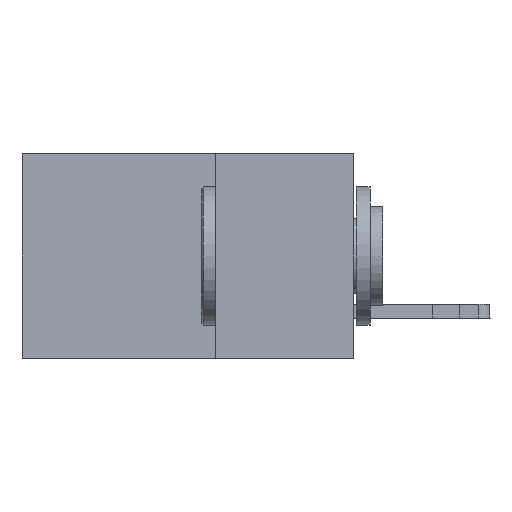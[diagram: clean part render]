
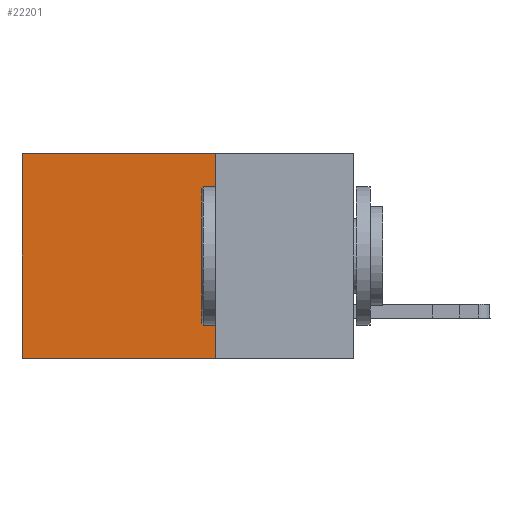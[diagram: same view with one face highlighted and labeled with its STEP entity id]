
A CAD part, left-side view. The second image highlights one B-rep face of the part: STEP entity #22201.
In plain terms, the highlighted planar face has unit normal (-1, 0, 0).
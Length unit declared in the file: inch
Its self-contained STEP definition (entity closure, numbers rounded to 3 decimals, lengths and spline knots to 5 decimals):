
#288 = DIRECTION ( 'NONE',  ( 0., 0., -1. ) ) ;
#457 = FACE_OUTER_BOUND ( 'NONE', #8507, .T. ) ;
#629 = LINE ( 'NONE', #10913, #10525 ) ;
#1062 = DIRECTION ( 'NONE',  ( 0., 0., -1. ) ) ;
#1547 = VERTEX_POINT ( 'NONE', #6921 ) ;
#2471 = ORIENTED_EDGE ( 'NONE', *, *, #16416, .F. ) ;
#4737 = DIRECTION ( 'NONE',  ( 0., 0., -1. ) ) ;
#6042 = EDGE_CURVE ( 'NONE', #14477, #6281, #6808, .T. ) ;
#6110 = CARTESIAN_POINT ( 'NONE',  ( 0.2875, 0.6, -0.37 ) ) ;
#6202 = VECTOR ( 'NONE', #288, 39.37008 ) ;
#6281 = VERTEX_POINT ( 'NONE', #16719 ) ;
#6305 = EDGE_CURVE ( 'NONE', #1547, #23799, #629, .T. ) ;
#6808 = LINE ( 'NONE', #19873, #6202 ) ;
#6815 = LINE ( 'NONE', #23169, #11470 ) ;
#6921 = CARTESIAN_POINT ( 'NONE',  ( 0.2875, 0.6, 0. ) ) ;
#7619 = LINE ( 'NONE', #21900, #17441 ) ;
#8507 = EDGE_LOOP ( 'NONE', ( #19367, #2471, #19189, #13010 ) ) ;
#10525 = VECTOR ( 'NONE', #1062, 39.37008 ) ;
#10913 = CARTESIAN_POINT ( 'NONE',  ( 0.2875, 0.6, 0. ) ) ;
#11470 = VECTOR ( 'NONE', #13450, 39.37008 ) ;
#12113 = DIRECTION ( 'NONE',  ( 0., 1., 0. ) ) ;
#13010 = ORIENTED_EDGE ( 'NONE', *, *, #20091, .T. ) ;
#13450 = DIRECTION ( 'NONE',  ( 0., 1., 0. ) ) ;
#14477 = VERTEX_POINT ( 'NONE', #16305 ) ;
#16305 = CARTESIAN_POINT ( 'NONE',  ( 0.2875, 0.25, 0. ) ) ;
#16416 = EDGE_CURVE ( 'NONE', #6281, #23799, #7619, .T. ) ;
#16514 = DIRECTION ( 'NONE',  ( 1., 0., 0. ) ) ;
#16719 = CARTESIAN_POINT ( 'NONE',  ( 0.2875, 0.25, -0.37 ) ) ;
#17441 = VECTOR ( 'NONE', #12113, 39.37008 ) ;
#18385 = AXIS2_PLACEMENT_3D ( 'NONE', #24222, #16514, #4737 ) ;
#19189 = ORIENTED_EDGE ( 'NONE', *, *, #6042, .F. ) ;
#19367 = ORIENTED_EDGE ( 'NONE', *, *, #6305, .T. ) ;
#19873 = CARTESIAN_POINT ( 'NONE',  ( 0.2875, 0.25, 0. ) ) ;
#20091 = EDGE_CURVE ( 'NONE', #14477, #1547, #6815, .T. ) ;
#21900 = CARTESIAN_POINT ( 'NONE',  ( 0.2875, 0.25, -0.37 ) ) ;
#22201 = ADVANCED_FACE ( 'NONE', ( #457 ), #22291, .F. ) ;
#22291 = PLANE ( 'NONE',  #18385 ) ;
#23169 = CARTESIAN_POINT ( 'NONE',  ( 0.2875, 0.25, 0. ) ) ;
#23799 = VERTEX_POINT ( 'NONE', #6110 ) ;
#24222 = CARTESIAN_POINT ( 'NONE',  ( 0.2875, 0.25, 0. ) ) ;
